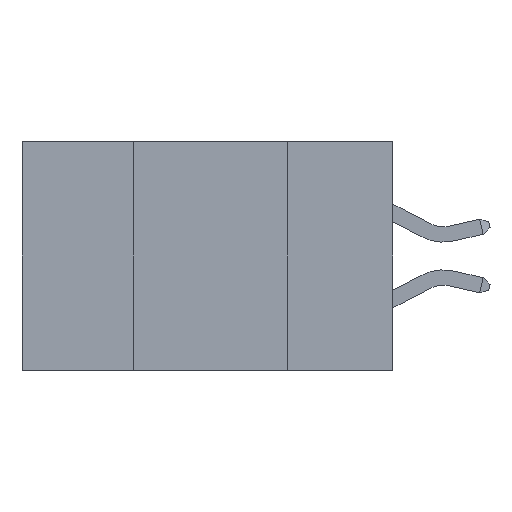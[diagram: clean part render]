
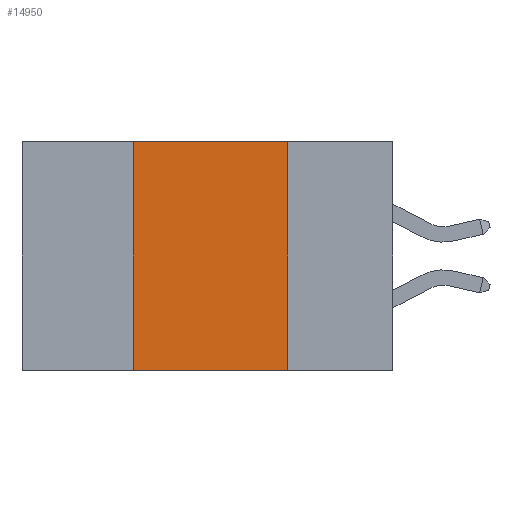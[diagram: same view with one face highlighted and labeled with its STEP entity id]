
A CAD part, left-side view. The second image highlights one B-rep face of the part: STEP entity #14950.
In plain terms, the highlighted planar face has unit normal (-1, 0, 0).
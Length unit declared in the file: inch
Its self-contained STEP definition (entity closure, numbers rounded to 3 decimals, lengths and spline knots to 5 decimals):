
#2913 = VECTOR ( 'NONE', #3497, 39.37008 ) ;
#3280 = ORIENTED_EDGE ( 'NONE', *, *, #36598, .F. ) ;
#3497 = DIRECTION ( 'NONE',  ( 0., 0., -1. ) ) ;
#5647 = VECTOR ( 'NONE', #21627, 39.37008 ) ;
#7540 = CARTESIAN_POINT ( 'NONE',  ( 0., 0.6, -0.37 ) ) ;
#7613 = AXIS2_PLACEMENT_3D ( 'NONE', #15133, #9121, #28605 ) ;
#9121 = DIRECTION ( 'NONE',  ( 1., 0., 0. ) ) ;
#10882 = VERTEX_POINT ( 'NONE', #22485 ) ;
#10884 = DIRECTION ( 'NONE',  ( 0., -1., 0. ) ) ;
#12792 = LINE ( 'NONE', #16959, #2913 ) ;
#12838 = LINE ( 'NONE', #24850, #42985 ) ;
#14950 = ADVANCED_FACE ( 'NONE', ( #32379 ), #31793, .F. ) ;
#15056 = ORIENTED_EDGE ( 'NONE', *, *, #42322, .F. ) ;
#15133 = CARTESIAN_POINT ( 'NONE',  ( 0., 0.6, 0. ) ) ;
#15608 = VERTEX_POINT ( 'NONE', #39694 ) ;
#16080 = ORIENTED_EDGE ( 'NONE', *, *, #34379, .T. ) ;
#16701 = LINE ( 'NONE', #7540, #31734 ) ;
#16959 = CARTESIAN_POINT ( 'NONE',  ( 0., 0.17, 0. ) ) ;
#17340 = VERTEX_POINT ( 'NONE', #31415 ) ;
#21627 = DIRECTION ( 'NONE',  ( 0., 0., 1. ) ) ;
#22485 = CARTESIAN_POINT ( 'NONE',  ( 0., 0.17, -0.37 ) ) ;
#23446 = EDGE_CURVE ( 'NONE', #33259, #17340, #37374, .T. ) ;
#24850 = CARTESIAN_POINT ( 'NONE',  ( 0., 0.6, 0. ) ) ;
#28134 = EDGE_LOOP ( 'NONE', ( #15056, #3280, #35840, #16080 ) ) ;
#28605 = DIRECTION ( 'NONE',  ( 0., 0., -1. ) ) ;
#31415 = CARTESIAN_POINT ( 'NONE',  ( 0., 0.42, 0. ) ) ;
#31734 = VECTOR ( 'NONE', #10884, 39.37008 ) ;
#31793 = PLANE ( 'NONE',  #7613 ) ;
#32379 = FACE_OUTER_BOUND ( 'NONE', #28134, .T. ) ;
#32761 = CARTESIAN_POINT ( 'NONE',  ( 0., 0.42, -0.37 ) ) ;
#33259 = VERTEX_POINT ( 'NONE', #32761 ) ;
#34379 = EDGE_CURVE ( 'NONE', #33259, #10882, #16701, .T. ) ;
#35840 = ORIENTED_EDGE ( 'NONE', *, *, #23446, .F. ) ;
#36598 = EDGE_CURVE ( 'NONE', #17340, #15608, #12838, .T. ) ;
#37374 = LINE ( 'NONE', #39505, #5647 ) ;
#37624 = DIRECTION ( 'NONE',  ( 0., -1., 0. ) ) ;
#39505 = CARTESIAN_POINT ( 'NONE',  ( 0., 0.42, 0. ) ) ;
#39694 = CARTESIAN_POINT ( 'NONE',  ( 0., 0.17, 0. ) ) ;
#42322 = EDGE_CURVE ( 'NONE', #15608, #10882, #12792, .T. ) ;
#42985 = VECTOR ( 'NONE', #37624, 39.37008 ) ;
